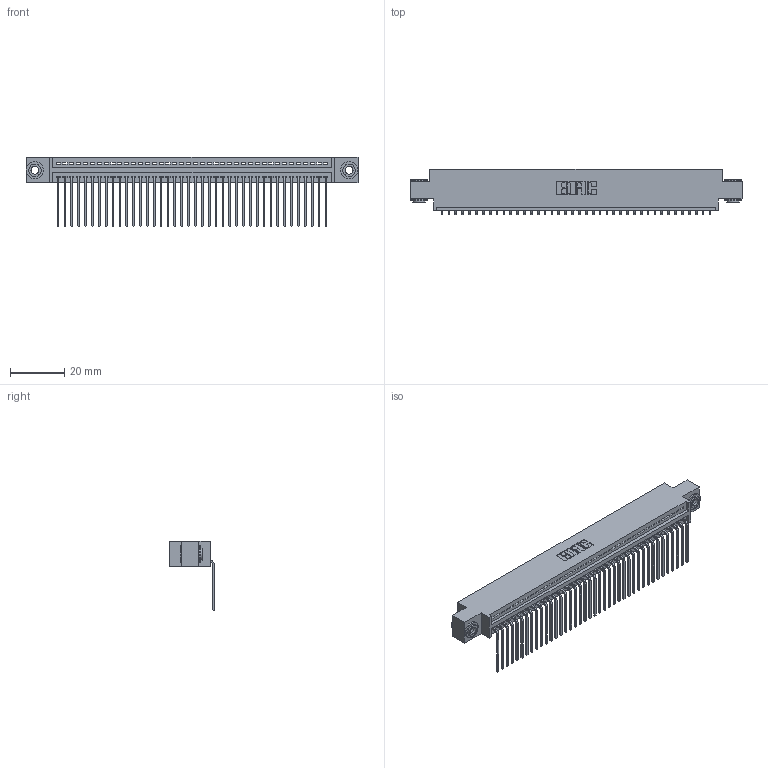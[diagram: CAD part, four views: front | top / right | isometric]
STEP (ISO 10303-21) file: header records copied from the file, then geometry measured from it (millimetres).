
FILE_DESCRIPTION (( 'STEP AP203' ), '1' );
FILE_NAME ('345-040-559-603.STEP', '2019-10-08T10:43:19', ( '' ), ( '' ), 'SwSTEP 2.0', 'SolidWorks 2016', '' );
FILE_SCHEMA (( 'CONFIG_CONTROL_DESIGN' ));
Length unit declared in the file: inch
Products named in the file (4): 345 Part_0.170 Offset - 0.156 Dia-TH; 345-292-001_558 559 Tail - 1; 345-040-559-603; 345-250-002_345-250-002-102
Assembly tree (43 placements, depth 2):
  345-040-559-603
    345 Part_0.170 Offset - 0.156 Dia-TH
    345-292-001_558 559 Tail - 1  x40
    345-250-002_345-250-002-102  x2
Bounding box: 122.81 x 16.75 x 25.53 mm (x, y, z)
Volume: 11687.4 mm3; surface area: 16628.5 mm2
Topology: 43 solids, 43 shells, 2568 faces, 7709 edges, 5082 vertices
Faces by surface type: plane 1774, cylinder 786, cone 8
Entity records: 31240 total; most frequent: CARTESIAN_POINT 5391, ORIENTED_EDGE 5358, DIRECTION 4741, EDGE_CURVE 2679, VECTOR 2363, LINE 2363, VERTEX_POINT 1782, AXIS2_PLACEMENT_3D 1189
